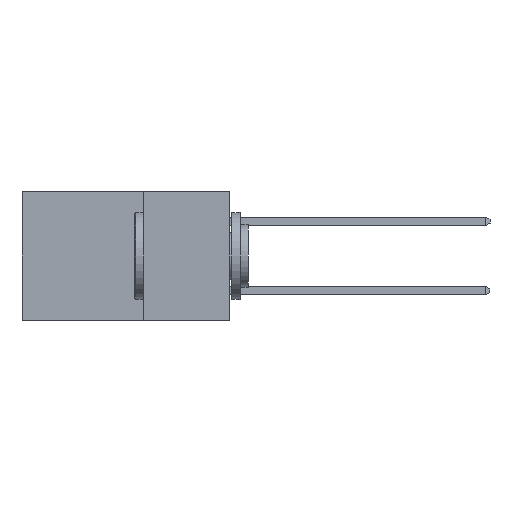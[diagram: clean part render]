
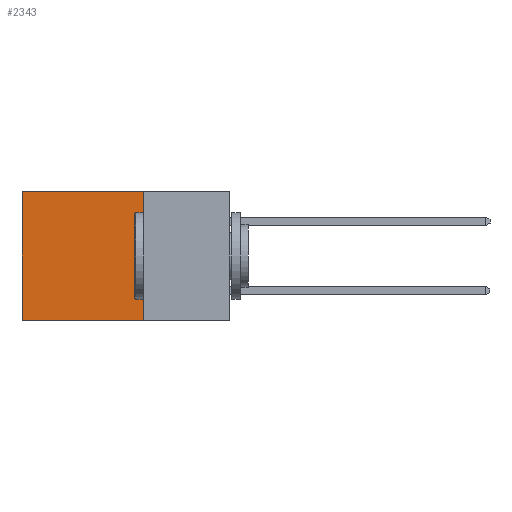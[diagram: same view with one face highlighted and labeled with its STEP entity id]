
A CAD part, left-side view. The second image highlights one B-rep face of the part: STEP entity #2343.
In plain terms, the highlighted planar face has unit normal (-1, 0, 0).
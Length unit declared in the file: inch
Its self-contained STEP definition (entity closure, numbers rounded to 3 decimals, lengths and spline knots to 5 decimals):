
#88 = VECTOR ( 'NONE', #13453, 39.37008 ) ;
#161 = CARTESIAN_POINT ( 'NONE',  ( 0.298, 0.6, -0.37 ) ) ;
#1859 = EDGE_CURVE ( 'NONE', #7917, #6602, #7491, .T. ) ;
#1936 = ORIENTED_EDGE ( 'NONE', *, *, #1859, .T. ) ;
#2146 = LINE ( 'NONE', #5718, #5411 ) ;
#2343 = ADVANCED_FACE ( 'NONE', ( #3330 ), #3351, .F. ) ;
#2928 = EDGE_CURVE ( 'NONE', #6602, #10933, #13662, .T. ) ;
#3139 = DIRECTION ( 'NONE',  ( 0., 0., -1. ) ) ;
#3330 = FACE_OUTER_BOUND ( 'NONE', #4774, .T. ) ;
#3351 = PLANE ( 'NONE',  #4960 ) ;
#4382 = CARTESIAN_POINT ( 'NONE',  ( 0.298, 0.25, 0. ) ) ;
#4671 = VECTOR ( 'NONE', #7052, 39.37008 ) ;
#4774 = EDGE_LOOP ( 'NONE', ( #9307, #7735, #9656, #1936 ) ) ;
#4960 = AXIS2_PLACEMENT_3D ( 'NONE', #16427, #17620, #17619 ) ;
#5411 = VECTOR ( 'NONE', #15331, 39.37008 ) ;
#5718 = CARTESIAN_POINT ( 'NONE',  ( 0.298, 0.25, 0. ) ) ;
#6602 = VERTEX_POINT ( 'NONE', #9040 ) ;
#6812 = VECTOR ( 'NONE', #3139, 39.37008 ) ;
#7052 = DIRECTION ( 'NONE',  ( 0., 1., 0. ) ) ;
#7491 = LINE ( 'NONE', #14309, #88 ) ;
#7735 = ORIENTED_EDGE ( 'NONE', *, *, #12281, .F. ) ;
#7917 = VERTEX_POINT ( 'NONE', #4382 ) ;
#9040 = CARTESIAN_POINT ( 'NONE',  ( 0.298, 0.6, 0. ) ) ;
#9307 = ORIENTED_EDGE ( 'NONE', *, *, #2928, .T. ) ;
#9656 = ORIENTED_EDGE ( 'NONE', *, *, #15684, .F. ) ;
#10130 = CARTESIAN_POINT ( 'NONE',  ( 0.298, 0.6, 0. ) ) ;
#10933 = VERTEX_POINT ( 'NONE', #161 ) ;
#11158 = CARTESIAN_POINT ( 'NONE',  ( 0.298, 0.25, -0.37 ) ) ;
#12281 = EDGE_CURVE ( 'NONE', #13799, #10933, #12535, .T. ) ;
#12535 = LINE ( 'NONE', #11158, #4671 ) ;
#13453 = DIRECTION ( 'NONE',  ( 0., 1., 0. ) ) ;
#13662 = LINE ( 'NONE', #10130, #6812 ) ;
#13799 = VERTEX_POINT ( 'NONE', #15753 ) ;
#14309 = CARTESIAN_POINT ( 'NONE',  ( 0.298, 0.25, 0. ) ) ;
#15331 = DIRECTION ( 'NONE',  ( 0., 0., -1. ) ) ;
#15684 = EDGE_CURVE ( 'NONE', #7917, #13799, #2146, .T. ) ;
#15753 = CARTESIAN_POINT ( 'NONE',  ( 0.298, 0.25, -0.37 ) ) ;
#16427 = CARTESIAN_POINT ( 'NONE',  ( 0.298, 0.25, 0. ) ) ;
#17619 = DIRECTION ( 'NONE',  ( 0., 0., -1. ) ) ;
#17620 = DIRECTION ( 'NONE',  ( 1., 0., 0. ) ) ;
